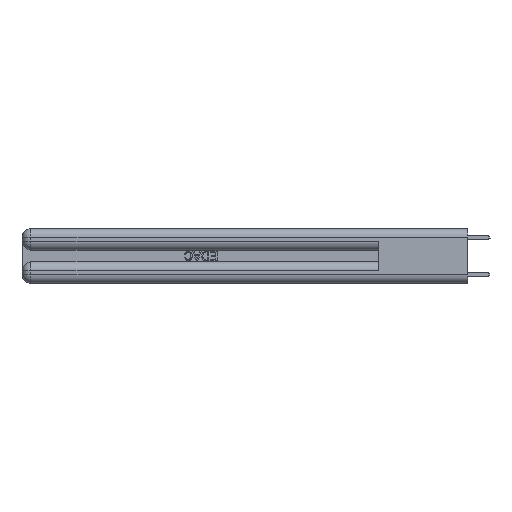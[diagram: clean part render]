
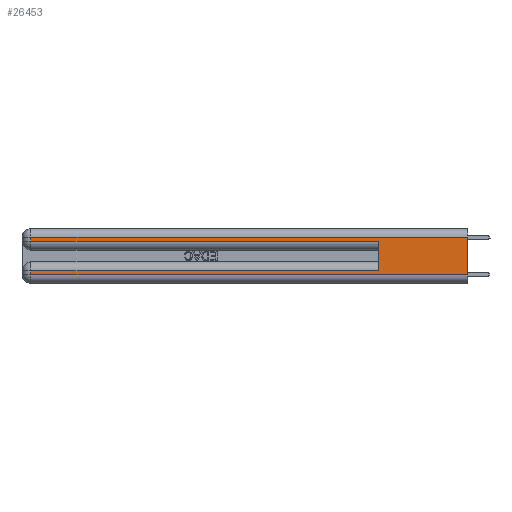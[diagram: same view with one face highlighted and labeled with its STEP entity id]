
A CAD part, left-side view. The second image highlights one B-rep face of the part: STEP entity #26453.
In plain terms, the highlighted planar face has unit normal (-1, 0, 0).
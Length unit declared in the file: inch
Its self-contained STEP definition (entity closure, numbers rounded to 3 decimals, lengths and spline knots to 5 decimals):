
#891 = VECTOR ( 'NONE', #11345, 39.37008 ) ;
#1669 = CARTESIAN_POINT ( 'NONE',  ( 0., 0., 0.285 ) ) ;
#2454 = CARTESIAN_POINT ( 'NONE',  ( 0., 0., 0.37 ) ) ;
#3405 = CARTESIAN_POINT ( 'NONE',  ( 0., 0.6, 0.145 ) ) ;
#3921 = EDGE_CURVE ( 'NONE', #22806, #11197, #12939, .T. ) ;
#4109 = DIRECTION ( 'NONE',  ( 0., 0., -1. ) ) ;
#4341 = ORIENTED_EDGE ( 'NONE', *, *, #30517, .T. ) ;
#4562 = CARTESIAN_POINT ( 'NONE',  ( 0., 2.94, 0.085 ) ) ;
#5341 = LINE ( 'NONE', #3405, #27247 ) ;
#5539 = VECTOR ( 'NONE', #28924, 39.37008 ) ;
#5681 = ORIENTED_EDGE ( 'NONE', *, *, #17048, .F. ) ;
#6271 = EDGE_CURVE ( 'NONE', #22806, #25005, #5341, .T. ) ;
#6691 = CARTESIAN_POINT ( 'NONE',  ( 0., 0.6, 0.285 ) ) ;
#8459 = DIRECTION ( 'NONE',  ( 0., 0., 1. ) ) ;
#10054 = ORIENTED_EDGE ( 'NONE', *, *, #6271, .F. ) ;
#10098 = DIRECTION ( 'NONE',  ( 0., -1., 0. ) ) ;
#10879 = VECTOR ( 'NONE', #21978, 39.37008 ) ;
#11039 = ORIENTED_EDGE ( 'NONE', *, *, #28490, .T. ) ;
#11197 = VERTEX_POINT ( 'NONE', #4562 ) ;
#11345 = DIRECTION ( 'NONE',  ( 0., 1., 0. ) ) ;
#11418 = CARTESIAN_POINT ( 'NONE',  ( 0., 2.94, 0.285 ) ) ;
#11677 = VERTEX_POINT ( 'NONE', #11418 ) ;
#11813 = DIRECTION ( 'NONE',  ( 1., 0., 0. ) ) ;
#12274 = CARTESIAN_POINT ( 'NONE',  ( 0., 0.6, 0.085 ) ) ;
#12939 = LINE ( 'NONE', #23713, #10879 ) ;
#13050 = CARTESIAN_POINT ( 'NONE',  ( 0., 2.94, 0.31 ) ) ;
#13264 = LINE ( 'NONE', #1669, #17413 ) ;
#13289 = VECTOR ( 'NONE', #16015, 39.37008 ) ;
#13363 = CARTESIAN_POINT ( 'NONE',  ( 0., 2.94, 0.37 ) ) ;
#14121 = CARTESIAN_POINT ( 'NONE',  ( 0., 0., 0.31 ) ) ;
#14921 = LINE ( 'NONE', #14121, #891 ) ;
#15386 = AXIS2_PLACEMENT_3D ( 'NONE', #32960, #11813, #4109 ) ;
#15764 = VERTEX_POINT ( 'NONE', #13050 ) ;
#16015 = DIRECTION ( 'NONE',  ( 0., 0., -1. ) ) ;
#16303 = LINE ( 'NONE', #18031, #17529 ) ;
#17048 = EDGE_CURVE ( 'NONE', #21199, #24111, #33617, .T. ) ;
#17413 = VECTOR ( 'NONE', #33406, 39.37008 ) ;
#17529 = VECTOR ( 'NONE', #10098, 39.37008 ) ;
#18029 = CARTESIAN_POINT ( 'NONE',  ( 0., 0., 0.31 ) ) ;
#18031 = CARTESIAN_POINT ( 'NONE',  ( 0., 0., 0.06 ) ) ;
#20021 = EDGE_LOOP ( 'NONE', ( #5681, #4341, #26724, #23081, #10054, #22558, #22322, #11039 ) ) ;
#21199 = VERTEX_POINT ( 'NONE', #18029 ) ;
#21231 = CARTESIAN_POINT ( 'NONE',  ( 0., 2.94, 0.06 ) ) ;
#21416 = LINE ( 'NONE', #24028, #28074 ) ;
#21819 = DIRECTION ( 'NONE',  ( 0., 0., -1. ) ) ;
#21978 = DIRECTION ( 'NONE',  ( 0., 1., 0. ) ) ;
#22322 = ORIENTED_EDGE ( 'NONE', *, *, #32750, .T. ) ;
#22558 = ORIENTED_EDGE ( 'NONE', *, *, #3921, .T. ) ;
#22761 = EDGE_CURVE ( 'NONE', #11677, #25005, #13264, .T. ) ;
#22806 = VERTEX_POINT ( 'NONE', #12274 ) ;
#22874 = LINE ( 'NONE', #13363, #13289 ) ;
#23081 = ORIENTED_EDGE ( 'NONE', *, *, #22761, .T. ) ;
#23713 = CARTESIAN_POINT ( 'NONE',  ( 0., 0., 0.085 ) ) ;
#23805 = FACE_OUTER_BOUND ( 'NONE', #20021, .T. ) ;
#24028 = CARTESIAN_POINT ( 'NONE',  ( 0., 2.94, 0.37 ) ) ;
#24111 = VERTEX_POINT ( 'NONE', #27914 ) ;
#25005 = VERTEX_POINT ( 'NONE', #6691 ) ;
#26453 = ADVANCED_FACE ( 'NONE', ( #23805 ), #27671, .F. ) ;
#26724 = ORIENTED_EDGE ( 'NONE', *, *, #29714, .T. ) ;
#27247 = VECTOR ( 'NONE', #8459, 39.37008 ) ;
#27671 = PLANE ( 'NONE',  #15386 ) ;
#27914 = CARTESIAN_POINT ( 'NONE',  ( 0., 0., 0.06 ) ) ;
#28074 = VECTOR ( 'NONE', #21819, 39.37008 ) ;
#28490 = EDGE_CURVE ( 'NONE', #32586, #24111, #16303, .T. ) ;
#28924 = DIRECTION ( 'NONE',  ( 0., 0., -1. ) ) ;
#29714 = EDGE_CURVE ( 'NONE', #15764, #11677, #22874, .T. ) ;
#30517 = EDGE_CURVE ( 'NONE', #21199, #15764, #14921, .T. ) ;
#32586 = VERTEX_POINT ( 'NONE', #21231 ) ;
#32750 = EDGE_CURVE ( 'NONE', #11197, #32586, #21416, .T. ) ;
#32960 = CARTESIAN_POINT ( 'NONE',  ( 0., 0., 0.37 ) ) ;
#33406 = DIRECTION ( 'NONE',  ( 0., -1., 0. ) ) ;
#33617 = LINE ( 'NONE', #2454, #5539 ) ;
